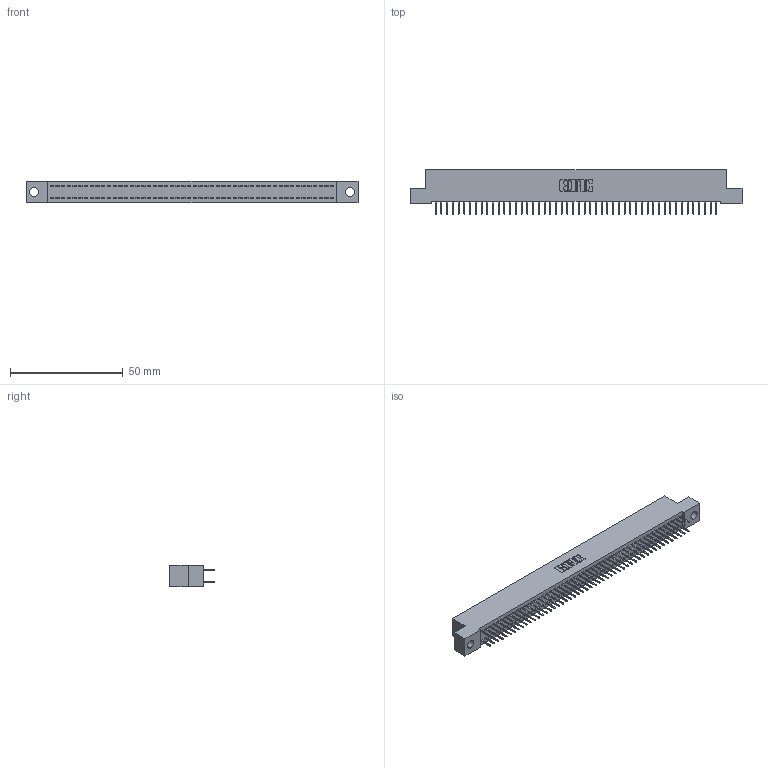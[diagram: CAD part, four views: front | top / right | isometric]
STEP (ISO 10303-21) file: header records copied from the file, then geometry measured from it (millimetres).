
FILE_DESCRIPTION (( 'STEP AP203' ), '1' );
FILE_NAME ('392-100-524-204.STEP', '2019-10-09T20:48:46', ( '' ), ( '' ), 'SwSTEP 2.0', 'SolidWorks 2016', '' );
FILE_SCHEMA (( 'CONFIG_CONTROL_DESIGN' ));
Length unit declared in the file: inch
Products named in the file (3): 342 Part_.156 TH; 345-292-001_345-293-124; 392-100-524-204
Assembly tree (101 placements, depth 2):
  392-100-524-204
    342 Part_.156 TH
    345-292-001_345-293-124  x100
Bounding box: 147.32 x 19.69 x 9.4 mm (x, y, z)
Volume: 13036.2 mm3; surface area: 20847.3 mm2
Topology: 101 solids, 101 shells, 5710 faces, 16199 edges, 10398 vertices
Faces by surface type: plane 4266, cylinder 1444
Entity records: 31077 total; most frequent: CARTESIAN_POINT 5138, ORIENTED_EDGE 5074, DIRECTION 4377, EDGE_CURVE 2537, VECTOR 2413, LINE 2413, VERTEX_POINT 1686, AXIS2_PLACEMENT_3D 982
